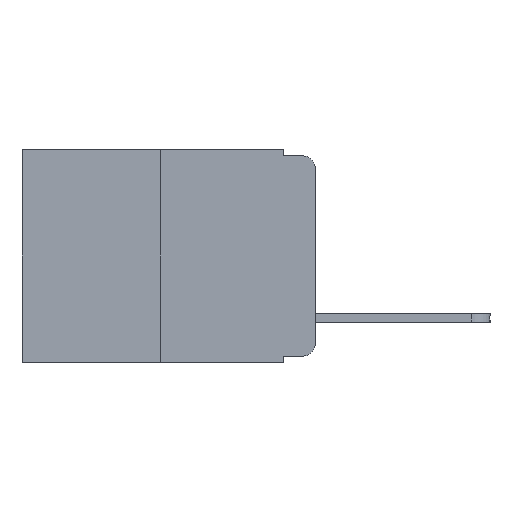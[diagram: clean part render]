
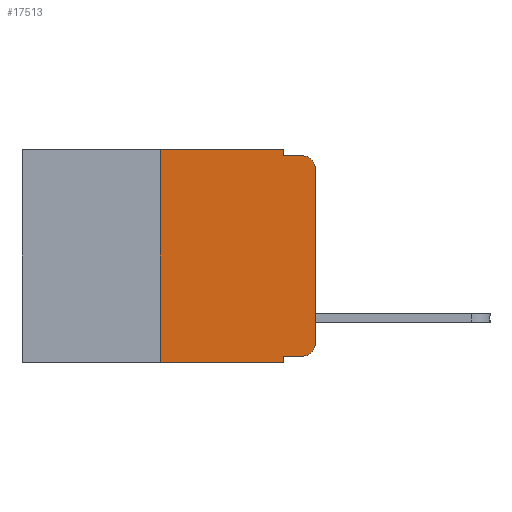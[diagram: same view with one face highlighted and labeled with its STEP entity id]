
A CAD part, left-side view. The second image highlights one B-rep face of the part: STEP entity #17513.
In plain terms, the highlighted planar face has unit normal (-1, 0, 0).
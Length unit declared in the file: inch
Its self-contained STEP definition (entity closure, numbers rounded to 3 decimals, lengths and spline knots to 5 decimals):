
#85 = CARTESIAN_POINT ( 'NONE',  ( 0., 0.051, -0.333 ) ) ;
#125 = ORIENTED_EDGE ( 'NONE', *, *, #16210, .T. ) ;
#185 = CARTESIAN_POINT ( 'NONE',  ( 0., 0., 0. ) ) ;
#409 = ORIENTED_EDGE ( 'NONE', *, *, #5613, .F. ) ;
#1065 = CARTESIAN_POINT ( 'NONE',  ( 0., 0.051, -0.01 ) ) ;
#1100 = DIRECTION ( 'NONE',  ( 0., -1., 0. ) ) ;
#1350 = EDGE_CURVE ( 'NONE', #17818, #20788, #11783, .T. ) ;
#1396 = CARTESIAN_POINT ( 'NONE',  ( 0., 0.473, -0.343 ) ) ;
#1817 = DIRECTION ( 'NONE',  ( 0., 0., -1. ) ) ;
#2514 = DIRECTION ( 'NONE',  ( 1., 0., 0. ) ) ;
#2744 = VECTOR ( 'NONE', #8904, 39.37008 ) ;
#2818 = LINE ( 'NONE', #5449, #11842 ) ;
#3633 = VERTEX_POINT ( 'NONE', #3784 ) ;
#3717 = DIRECTION ( 'NONE',  ( -1., 0., 0. ) ) ;
#3784 = CARTESIAN_POINT ( 'NONE',  ( 0., 0.25, -0.343 ) ) ;
#4282 = VERTEX_POINT ( 'NONE', #6050 ) ;
#4400 = VECTOR ( 'NONE', #18490, 39.37008 ) ;
#4408 = VECTOR ( 'NONE', #1100, 39.37008 ) ;
#4422 = DIRECTION ( 'NONE',  ( -1., 0., 0. ) ) ;
#4447 = ORIENTED_EDGE ( 'NONE', *, *, #13135, .F. ) ;
#4603 = EDGE_CURVE ( 'NONE', #19636, #10110, #9514, .T. ) ;
#4777 = ORIENTED_EDGE ( 'NONE', *, *, #9597, .T. ) ;
#4940 = DIRECTION ( 'NONE',  ( 0., -1., 0. ) ) ;
#4994 = VECTOR ( 'NONE', #7313, 39.37008 ) ;
#5327 = AXIS2_PLACEMENT_3D ( 'NONE', #14404, #4422, #16056 ) ;
#5449 = CARTESIAN_POINT ( 'NONE',  ( 0., 0.051, 0. ) ) ;
#5613 = EDGE_CURVE ( 'NONE', #3633, #8016, #13305, .T. ) ;
#5843 = PLANE ( 'NONE',  #10818 ) ;
#6050 = CARTESIAN_POINT ( 'NONE',  ( 0., 0.02, -0.01 ) ) ;
#7137 = VECTOR ( 'NONE', #4940, 39.37008 ) ;
#7313 = DIRECTION ( 'NONE',  ( 0., -1., 0. ) ) ;
#7724 = CARTESIAN_POINT ( 'NONE',  ( 0., 0.02, -0.333 ) ) ;
#7960 = EDGE_CURVE ( 'NONE', #3633, #11218, #10468, .T. ) ;
#8016 = VERTEX_POINT ( 'NONE', #13415 ) ;
#8255 = ORIENTED_EDGE ( 'NONE', *, *, #8725, .F. ) ;
#8623 = VECTOR ( 'NONE', #1817, 39.37008 ) ;
#8725 = EDGE_CURVE ( 'NONE', #12404, #10192, #17329, .T. ) ;
#8904 = DIRECTION ( 'NONE',  ( 0., 0., 1. ) ) ;
#9514 = LINE ( 'NONE', #21554, #4994 ) ;
#9597 = EDGE_CURVE ( 'NONE', #10110, #17818, #17809, .T. ) ;
#9969 = CARTESIAN_POINT ( 'NONE',  ( 0., 0.051, -0.343 ) ) ;
#10110 = VERTEX_POINT ( 'NONE', #7724 ) ;
#10192 = VERTEX_POINT ( 'NONE', #1065 ) ;
#10326 = CIRCLE ( 'NONE', #13908, 0.02 ) ;
#10397 = CARTESIAN_POINT ( 'NONE',  ( 0., 0.051, 0. ) ) ;
#10468 = LINE ( 'NONE', #1396, #14280 ) ;
#10818 = AXIS2_PLACEMENT_3D ( 'NONE', #14221, #2514, #14285 ) ;
#11061 = LINE ( 'NONE', #14879, #7137 ) ;
#11218 = VERTEX_POINT ( 'NONE', #9969 ) ;
#11783 = LINE ( 'NONE', #185, #2744 ) ;
#11842 = VECTOR ( 'NONE', #16989, 39.37008 ) ;
#11933 = EDGE_CURVE ( 'NONE', #19636, #11218, #2818, .T. ) ;
#12404 = VERTEX_POINT ( 'NONE', #18920 ) ;
#12948 = FACE_OUTER_BOUND ( 'NONE', #13290, .T. ) ;
#13135 = EDGE_CURVE ( 'NONE', #10192, #4282, #17669, .T. ) ;
#13283 = DIRECTION ( 'NONE',  ( 0., -1., 0. ) ) ;
#13290 = EDGE_LOOP ( 'NONE', ( #18651, #125, #4447, #8255, #19685, #409, #19413, #16305, #15917, #4777 ) ) ;
#13305 = LINE ( 'NONE', #16832, #4400 ) ;
#13415 = CARTESIAN_POINT ( 'NONE',  ( 0., 0.25, 0. ) ) ;
#13768 = CARTESIAN_POINT ( 'NONE',  ( 0., 0.02, -0.03 ) ) ;
#13908 = AXIS2_PLACEMENT_3D ( 'NONE', #13768, #3717, #15394 ) ;
#14221 = CARTESIAN_POINT ( 'NONE',  ( 0., 0.473, 0. ) ) ;
#14280 = VECTOR ( 'NONE', #13283, 39.37008 ) ;
#14285 = DIRECTION ( 'NONE',  ( 0., 0., -1. ) ) ;
#14404 = CARTESIAN_POINT ( 'NONE',  ( 0., 0.02, -0.313 ) ) ;
#14879 = CARTESIAN_POINT ( 'NONE',  ( 0., 0.473, 0. ) ) ;
#15394 = DIRECTION ( 'NONE',  ( 0., 0., -1. ) ) ;
#15567 = CARTESIAN_POINT ( 'NONE',  ( 0., 0., -0.03 ) ) ;
#15917 = ORIENTED_EDGE ( 'NONE', *, *, #4603, .T. ) ;
#16056 = DIRECTION ( 'NONE',  ( 0., 0., -1. ) ) ;
#16210 = EDGE_CURVE ( 'NONE', #20788, #4282, #10326, .T. ) ;
#16305 = ORIENTED_EDGE ( 'NONE', *, *, #11933, .F. ) ;
#16832 = CARTESIAN_POINT ( 'NONE',  ( 0., 0.25, 0. ) ) ;
#16989 = DIRECTION ( 'NONE',  ( 0., 0., -1. ) ) ;
#17329 = LINE ( 'NONE', #10397, #8623 ) ;
#17513 = ADVANCED_FACE ( 'NONE', ( #12948 ), #5843, .F. ) ;
#17669 = LINE ( 'NONE', #21178, #4408 ) ;
#17809 = CIRCLE ( 'NONE', #5327, 0.02 ) ;
#17818 = VERTEX_POINT ( 'NONE', #18011 ) ;
#18011 = CARTESIAN_POINT ( 'NONE',  ( 0., 0., -0.313 ) ) ;
#18490 = DIRECTION ( 'NONE',  ( 0., 0., 1. ) ) ;
#18651 = ORIENTED_EDGE ( 'NONE', *, *, #1350, .T. ) ;
#18920 = CARTESIAN_POINT ( 'NONE',  ( 0., 0.051, 0. ) ) ;
#19413 = ORIENTED_EDGE ( 'NONE', *, *, #7960, .T. ) ;
#19455 = EDGE_CURVE ( 'NONE', #8016, #12404, #11061, .T. ) ;
#19636 = VERTEX_POINT ( 'NONE', #85 ) ;
#19685 = ORIENTED_EDGE ( 'NONE', *, *, #19455, .F. ) ;
#20788 = VERTEX_POINT ( 'NONE', #15567 ) ;
#21178 = CARTESIAN_POINT ( 'NONE',  ( 0., 0.051, -0.01 ) ) ;
#21554 = CARTESIAN_POINT ( 'NONE',  ( 0., 0.051, -0.333 ) ) ;
